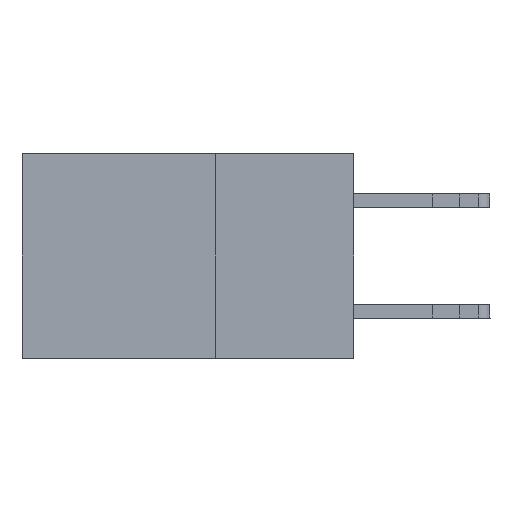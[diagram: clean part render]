
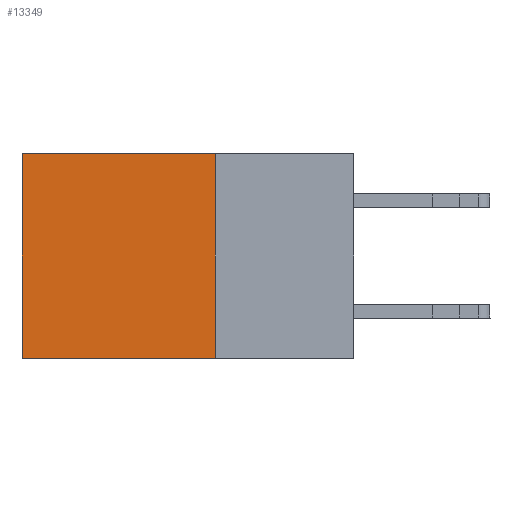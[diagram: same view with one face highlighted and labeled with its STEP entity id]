
A CAD part, left-side view. The second image highlights one B-rep face of the part: STEP entity #13349.
In plain terms, the highlighted planar face has unit normal (-1, 0, 0).
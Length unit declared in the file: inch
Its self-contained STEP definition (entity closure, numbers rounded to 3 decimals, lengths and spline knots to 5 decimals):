
#2510 = DIRECTION ( 'NONE',  ( 0., 0., -1. ) ) ;
#2632 = CARTESIAN_POINT ( 'NONE',  ( 0.2875, 0.6, -0.37 ) ) ;
#3242 = LINE ( 'NONE', #4689, #8586 ) ;
#4145 = EDGE_CURVE ( 'NONE', #12410, #13143, #20578, .T. ) ;
#4689 = CARTESIAN_POINT ( 'NONE',  ( 0.2875, 0.6, 0. ) ) ;
#5420 = CARTESIAN_POINT ( 'NONE',  ( 0.2875, 0.6, 0. ) ) ;
#5597 = ORIENTED_EDGE ( 'NONE', *, *, #12991, .T. ) ;
#6171 = ORIENTED_EDGE ( 'NONE', *, *, #21533, .T. ) ;
#7326 = LINE ( 'NONE', #15357, #8731 ) ;
#8457 = DIRECTION ( 'NONE',  ( 0., 1., 0. ) ) ;
#8586 = VECTOR ( 'NONE', #19981, 39.37008 ) ;
#8731 = VECTOR ( 'NONE', #13922, 39.37008 ) ;
#9631 = DIRECTION ( 'NONE',  ( 1., 0., 0. ) ) ;
#10928 = CARTESIAN_POINT ( 'NONE',  ( 0.2875, 0.25, -0.37 ) ) ;
#11500 = FACE_OUTER_BOUND ( 'NONE', #14584, .T. ) ;
#12164 = ORIENTED_EDGE ( 'NONE', *, *, #14427, .F. ) ;
#12410 = VERTEX_POINT ( 'NONE', #21150 ) ;
#12855 = VERTEX_POINT ( 'NONE', #2632 ) ;
#12930 = PLANE ( 'NONE',  #13662 ) ;
#12991 = EDGE_CURVE ( 'NONE', #12410, #20363, #7326, .T. ) ;
#13143 = VERTEX_POINT ( 'NONE', #10928 ) ;
#13349 = ADVANCED_FACE ( 'NONE', ( #11500 ), #12930, .F. ) ;
#13383 = ORIENTED_EDGE ( 'NONE', *, *, #4145, .F. ) ;
#13662 = AXIS2_PLACEMENT_3D ( 'NONE', #17977, #9631, #15024 ) ;
#13922 = DIRECTION ( 'NONE',  ( 0., 1., 0. ) ) ;
#13972 = CARTESIAN_POINT ( 'NONE',  ( 0.2875, 0.25, 0. ) ) ;
#14427 = EDGE_CURVE ( 'NONE', #13143, #12855, #18449, .T. ) ;
#14584 = EDGE_LOOP ( 'NONE', ( #6171, #12164, #13383, #5597 ) ) ;
#15024 = DIRECTION ( 'NONE',  ( 0., 0., -1. ) ) ;
#15357 = CARTESIAN_POINT ( 'NONE',  ( 0.2875, 0.25, 0. ) ) ;
#16834 = CARTESIAN_POINT ( 'NONE',  ( 0.2875, 0.25, -0.37 ) ) ;
#17977 = CARTESIAN_POINT ( 'NONE',  ( 0.2875, 0.25, 0. ) ) ;
#18449 = LINE ( 'NONE', #16834, #18676 ) ;
#18676 = VECTOR ( 'NONE', #8457, 39.37008 ) ;
#18823 = VECTOR ( 'NONE', #2510, 39.37008 ) ;
#19981 = DIRECTION ( 'NONE',  ( 0., 0., -1. ) ) ;
#20363 = VERTEX_POINT ( 'NONE', #5420 ) ;
#20578 = LINE ( 'NONE', #13972, #18823 ) ;
#21150 = CARTESIAN_POINT ( 'NONE',  ( 0.2875, 0.25, 0. ) ) ;
#21533 = EDGE_CURVE ( 'NONE', #20363, #12855, #3242, .T. ) ;
